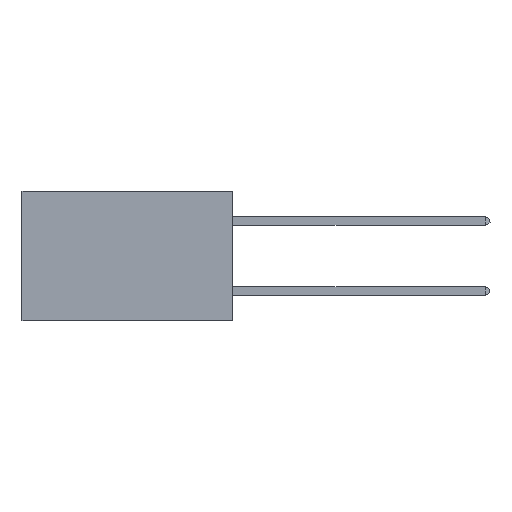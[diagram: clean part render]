
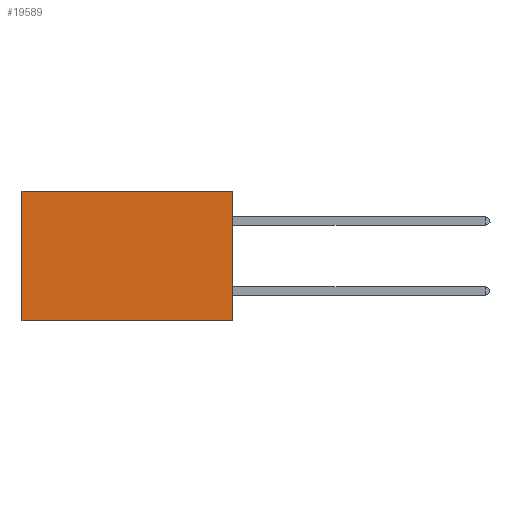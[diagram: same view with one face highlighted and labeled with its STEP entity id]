
A CAD part, left-side view. The second image highlights one B-rep face of the part: STEP entity #19589.
In plain terms, the highlighted planar face has unit normal (-1, 0, 0).
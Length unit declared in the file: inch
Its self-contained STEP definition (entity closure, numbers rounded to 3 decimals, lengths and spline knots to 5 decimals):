
#4130 = VECTOR ( 'NONE', #35125, 39.37008 ) ;
#4425 = FACE_OUTER_BOUND ( 'NONE', #25339, .T. ) ;
#4924 = VECTOR ( 'NONE', #11446, 39.37008 ) ;
#6956 = CARTESIAN_POINT ( 'NONE',  ( 0.2875, 0.6, 0. ) ) ;
#7457 = DIRECTION ( 'NONE',  ( 0., 1., 0. ) ) ;
#8251 = ORIENTED_EDGE ( 'NONE', *, *, #26457, .F. ) ;
#8559 = EDGE_CURVE ( 'NONE', #13519, #37075, #43718, .T. ) ;
#8940 = VERTEX_POINT ( 'NONE', #11858 ) ;
#9951 = ORIENTED_EDGE ( 'NONE', *, *, #8559, .T. ) ;
#11446 = DIRECTION ( 'NONE',  ( 0., 1., 0. ) ) ;
#11790 = CARTESIAN_POINT ( 'NONE',  ( 0.2875, 0., 0. ) ) ;
#11858 = CARTESIAN_POINT ( 'NONE',  ( 0.2875, 0., -0.37 ) ) ;
#13304 = CARTESIAN_POINT ( 'NONE',  ( 0.2875, 0.6, 0. ) ) ;
#13519 = VERTEX_POINT ( 'NONE', #6956 ) ;
#14412 = LINE ( 'NONE', #36261, #4924 ) ;
#17074 = ORIENTED_EDGE ( 'NONE', *, *, #24388, .T. ) ;
#18238 = DIRECTION ( 'NONE',  ( 0., 0., -1. ) ) ;
#19589 = ADVANCED_FACE ( 'NONE', ( #4425 ), #44502, .F. ) ;
#23246 = DIRECTION ( 'NONE',  ( 1., 0., 0. ) ) ;
#24388 = EDGE_CURVE ( 'NONE', #39624, #13519, #29151, .T. ) ;
#25339 = EDGE_LOOP ( 'NONE', ( #9951, #8251, #43779, #17074 ) ) ;
#25822 = VECTOR ( 'NONE', #7457, 39.37008 ) ;
#26457 = EDGE_CURVE ( 'NONE', #8940, #37075, #14412, .T. ) ;
#28702 = VECTOR ( 'NONE', #18238, 39.37008 ) ;
#29151 = LINE ( 'NONE', #31784, #25822 ) ;
#30070 = DIRECTION ( 'NONE',  ( 0., 0., -1. ) ) ;
#31784 = CARTESIAN_POINT ( 'NONE',  ( 0.2875, 0., 0. ) ) ;
#33377 = CARTESIAN_POINT ( 'NONE',  ( 0.2875, 0.6, -0.37 ) ) ;
#34802 = AXIS2_PLACEMENT_3D ( 'NONE', #11790, #23246, #30070 ) ;
#35125 = DIRECTION ( 'NONE',  ( 0., 0., -1. ) ) ;
#36261 = CARTESIAN_POINT ( 'NONE',  ( 0.2875, 0., -0.37 ) ) ;
#37075 = VERTEX_POINT ( 'NONE', #33377 ) ;
#39527 = EDGE_CURVE ( 'NONE', #39624, #8940, #45367, .T. ) ;
#39574 = CARTESIAN_POINT ( 'NONE',  ( 0.2875, 0., 0. ) ) ;
#39624 = VERTEX_POINT ( 'NONE', #45756 ) ;
#43718 = LINE ( 'NONE', #13304, #4130 ) ;
#43779 = ORIENTED_EDGE ( 'NONE', *, *, #39527, .F. ) ;
#44502 = PLANE ( 'NONE',  #34802 ) ;
#45367 = LINE ( 'NONE', #39574, #28702 ) ;
#45756 = CARTESIAN_POINT ( 'NONE',  ( 0.2875, 0., 0. ) ) ;
